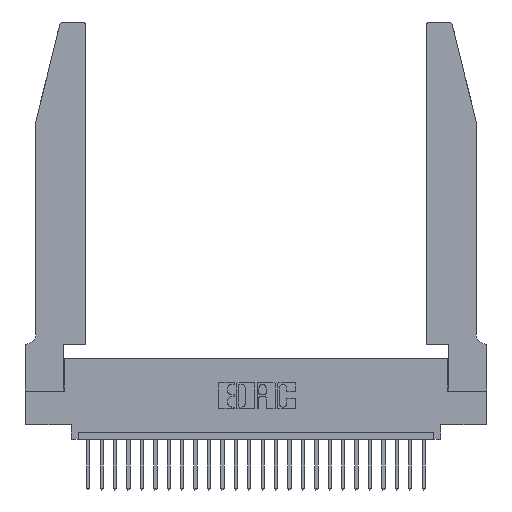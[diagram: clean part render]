
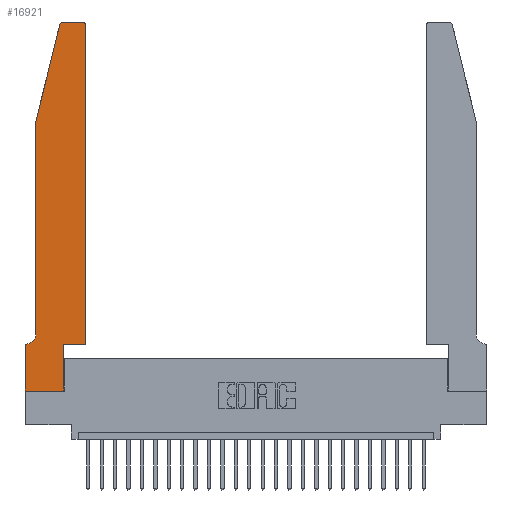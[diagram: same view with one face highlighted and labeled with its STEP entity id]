
A CAD part, top view. The second image highlights one B-rep face of the part: STEP entity #16921.
In plain terms, the highlighted planar face has unit normal (0, 0, 1).
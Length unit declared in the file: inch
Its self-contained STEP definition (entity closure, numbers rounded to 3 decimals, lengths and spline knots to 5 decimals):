
#134 = CIRCLE ( 'NONE', #18788, 0.03 ) ;
#267 = ORIENTED_EDGE ( 'NONE', *, *, #10824, .T. ) ;
#732 = AXIS2_PLACEMENT_3D ( 'NONE', #14484, #24806, #22666 ) ;
#791 = EDGE_CURVE ( 'NONE', #959, #16089, #4728, .T. ) ;
#959 = VERTEX_POINT ( 'NONE', #5390 ) ;
#1065 = DIRECTION ( 'NONE',  ( -1., 0., 0. ) ) ;
#1127 = VERTEX_POINT ( 'NONE', #17424 ) ;
#1224 = EDGE_CURVE ( 'NONE', #22051, #19494, #17575, .T. ) ;
#1327 = LINE ( 'NONE', #9141, #20291 ) ;
#1813 = CARTESIAN_POINT ( 'NONE',  ( 0.4205, 2.72, 0.37 ) ) ;
#2155 = ORIENTED_EDGE ( 'NONE', *, *, #20305, .T. ) ;
#2986 = LINE ( 'NONE', #14616, #5237 ) ;
#3015 = ORIENTED_EDGE ( 'NONE', *, *, #3953, .T. ) ;
#3058 = ORIENTED_EDGE ( 'NONE', *, *, #24258, .T. ) ;
#3169 = CARTESIAN_POINT ( 'NONE',  ( 0., 0., 0.37 ) ) ;
#3216 = VECTOR ( 'NONE', #19354, 39.37008 ) ;
#3953 = EDGE_CURVE ( 'NONE', #23507, #8753, #18114, .T. ) ;
#4174 = LINE ( 'NONE', #11388, #21827 ) ;
#4182 = DIRECTION ( 'NONE',  ( 1., 0., 0. ) ) ;
#4433 = EDGE_CURVE ( 'NONE', #19494, #8410, #1327, .T. ) ;
#4728 = CIRCLE ( 'NONE', #732, 0.07 ) ;
#4749 = DIRECTION ( 'NONE',  ( 1., 0., 0. ) ) ;
#5097 = ORIENTED_EDGE ( 'NONE', *, *, #4433, .T. ) ;
#5237 = VECTOR ( 'NONE', #8429, 39.37008 ) ;
#5390 = CARTESIAN_POINT ( 'NONE',  ( 0.0755, 0.42, 0.37 ) ) ;
#5669 = CARTESIAN_POINT ( 'NONE',  ( 0.2605, 2.75, 0.37 ) ) ;
#5793 = CARTESIAN_POINT ( 'NONE',  ( 0.2865, 0.35, 0.37 ) ) ;
#6346 = EDGE_CURVE ( 'NONE', #8410, #23507, #25014, .T. ) ;
#6382 = CARTESIAN_POINT ( 'NONE',  ( 0.0755, 2., 0.37 ) ) ;
#6806 = LINE ( 'NONE', #23049, #17064 ) ;
#7295 = FACE_OUTER_BOUND ( 'NONE', #17509, .T. ) ;
#7527 = ORIENTED_EDGE ( 'NONE', *, *, #1224, .T. ) ;
#8410 = VERTEX_POINT ( 'NONE', #19136 ) ;
#8429 = DIRECTION ( 'NONE',  ( 0., -1., 0. ) ) ;
#8439 = DIRECTION ( 'NONE',  ( 0., 0., 1. ) ) ;
#8456 = ORIENTED_EDGE ( 'NONE', *, *, #6346, .T. ) ;
#8753 = VERTEX_POINT ( 'NONE', #22191 ) ;
#8925 = EDGE_CURVE ( 'NONE', #15845, #14926, #134, .T. ) ;
#9141 = CARTESIAN_POINT ( 'NONE',  ( 0.4505, 0.35, 0.37 ) ) ;
#9162 = DIRECTION ( 'NONE',  ( -0.239, -0.971, 0. ) ) ;
#10040 = CARTESIAN_POINT ( 'NONE',  ( 0.284, 2.72, 0.37 ) ) ;
#10178 = DIRECTION ( 'NONE',  ( 0., 0., 1. ) ) ;
#10344 = CARTESIAN_POINT ( 'NONE',  ( 0.25487, 2.72718, 0.37 ) ) ;
#10403 = CARTESIAN_POINT ( 'NONE',  ( 0.4505, 2.72, 0.37 ) ) ;
#10454 = CARTESIAN_POINT ( 'NONE',  ( 0., 0.35, 0.37 ) ) ;
#10633 = AXIS2_PLACEMENT_3D ( 'NONE', #1813, #10178, #4182 ) ;
#10824 = EDGE_CURVE ( 'NONE', #18934, #22051, #19690, .T. ) ;
#10865 = ORIENTED_EDGE ( 'NONE', *, *, #791, .T. ) ;
#11021 = VECTOR ( 'NONE', #12601, 39.37008 ) ;
#11028 = ORIENTED_EDGE ( 'NONE', *, *, #14089, .T. ) ;
#11388 = CARTESIAN_POINT ( 'NONE',  ( 0.0755, 0.35, 0.37 ) ) ;
#11829 = CARTESIAN_POINT ( 'NONE',  ( 0.284, 2.75, 0.37 ) ) ;
#12601 = DIRECTION ( 'NONE',  ( 0., -1., 0. ) ) ;
#13061 = CARTESIAN_POINT ( 'NONE',  ( 0.2865, 0., 0.37 ) ) ;
#13186 = CARTESIAN_POINT ( 'NONE',  ( 0.4505, 0.35, 0.37 ) ) ;
#14089 = EDGE_CURVE ( 'NONE', #1127, #959, #15155, .T. ) ;
#14484 = CARTESIAN_POINT ( 'NONE',  ( 0.0055, 0.42, 0.37 ) ) ;
#14616 = CARTESIAN_POINT ( 'NONE',  ( 0., 0., 0.37 ) ) ;
#14737 = EDGE_CURVE ( 'NONE', #8753, #15845, #22093, .T. ) ;
#14926 = VERTEX_POINT ( 'NONE', #10344 ) ;
#15155 = LINE ( 'NONE', #6382, #11021 ) ;
#15845 = VERTEX_POINT ( 'NONE', #11829 ) ;
#16089 = VERTEX_POINT ( 'NONE', #16917 ) ;
#16455 = VECTOR ( 'NONE', #4749, 39.37008 ) ;
#16867 = DIRECTION ( 'NONE',  ( 1., 0., 0. ) ) ;
#16917 = CARTESIAN_POINT ( 'NONE',  ( 0.0055, 0.35, 0.37 ) ) ;
#16921 = ADVANCED_FACE ( 'NONE', ( #7295 ), #19014, .T. ) ;
#17000 = ORIENTED_EDGE ( 'NONE', *, *, #14737, .T. ) ;
#17064 = VECTOR ( 'NONE', #9162, 39.37008 ) ;
#17424 = CARTESIAN_POINT ( 'NONE',  ( 0.0755, 2., 0.37 ) ) ;
#17509 = EDGE_LOOP ( 'NONE', ( #17000, #24302, #3058, #11028, #10865, #23016, #2155, #267, #7527, #5097, #8456, #3015 ) ) ;
#17575 = LINE ( 'NONE', #5793, #23265 ) ;
#18096 = DIRECTION ( 'NONE',  ( 1., 0., 0. ) ) ;
#18114 = CIRCLE ( 'NONE', #10633, 0.03 ) ;
#18641 = VECTOR ( 'NONE', #24090, 39.37008 ) ;
#18788 = AXIS2_PLACEMENT_3D ( 'NONE', #10040, #20128, #18096 ) ;
#18934 = VERTEX_POINT ( 'NONE', #21244 ) ;
#19014 = PLANE ( 'NONE',  #20004 ) ;
#19136 = CARTESIAN_POINT ( 'NONE',  ( 0.4505, 0.35, 0.37 ) ) ;
#19354 = DIRECTION ( 'NONE',  ( 0., 1., 0. ) ) ;
#19375 = CARTESIAN_POINT ( 'NONE',  ( 0.2865, 0.35, 0.37 ) ) ;
#19494 = VERTEX_POINT ( 'NONE', #19375 ) ;
#19690 = LINE ( 'NONE', #3169, #16455 ) ;
#20004 = AXIS2_PLACEMENT_3D ( 'NONE', #22802, #8439, #16867 ) ;
#20128 = DIRECTION ( 'NONE',  ( 0., 0., 1. ) ) ;
#20144 = DIRECTION ( 'NONE',  ( 0., 1., 0. ) ) ;
#20291 = VECTOR ( 'NONE', #22607, 39.37008 ) ;
#20305 = EDGE_CURVE ( 'NONE', #22554, #18934, #2986, .T. ) ;
#21244 = CARTESIAN_POINT ( 'NONE',  ( 0., 0., 0.37 ) ) ;
#21827 = VECTOR ( 'NONE', #1065, 39.37008 ) ;
#22051 = VERTEX_POINT ( 'NONE', #13061 ) ;
#22093 = LINE ( 'NONE', #5669, #18641 ) ;
#22141 = EDGE_CURVE ( 'NONE', #16089, #22554, #4174, .T. ) ;
#22191 = CARTESIAN_POINT ( 'NONE',  ( 0.4205, 2.75, 0.37 ) ) ;
#22554 = VERTEX_POINT ( 'NONE', #10454 ) ;
#22607 = DIRECTION ( 'NONE',  ( 1., 0., 0. ) ) ;
#22666 = DIRECTION ( 'NONE',  ( -1., 0., 0. ) ) ;
#22802 = CARTESIAN_POINT ( 'NONE',  ( 0., 0.35, 0.37 ) ) ;
#23016 = ORIENTED_EDGE ( 'NONE', *, *, #22141, .T. ) ;
#23049 = CARTESIAN_POINT ( 'NONE',  ( 0.0755, 2., 0.37 ) ) ;
#23265 = VECTOR ( 'NONE', #20144, 39.37008 ) ;
#23507 = VERTEX_POINT ( 'NONE', #10403 ) ;
#24090 = DIRECTION ( 'NONE',  ( -1., 0., 0. ) ) ;
#24258 = EDGE_CURVE ( 'NONE', #14926, #1127, #6806, .T. ) ;
#24302 = ORIENTED_EDGE ( 'NONE', *, *, #8925, .T. ) ;
#24806 = DIRECTION ( 'NONE',  ( 0., 0., -1. ) ) ;
#25014 = LINE ( 'NONE', #13186, #3216 ) ;
